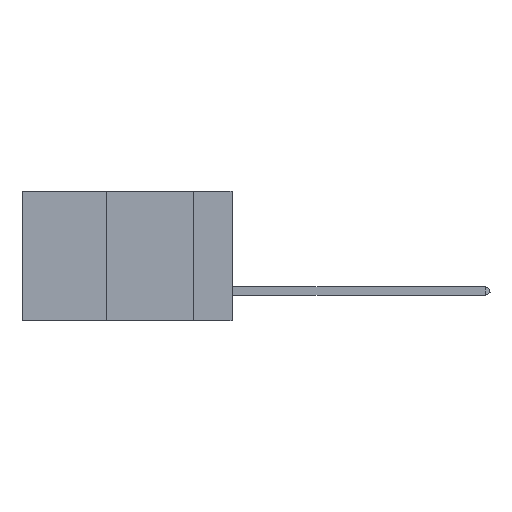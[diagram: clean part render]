
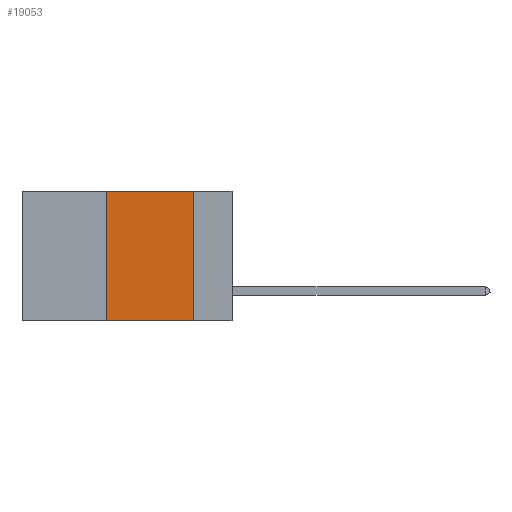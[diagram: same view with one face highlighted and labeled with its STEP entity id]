
A CAD part, left-side view. The second image highlights one B-rep face of the part: STEP entity #19053.
In plain terms, the highlighted planar face has unit normal (-1, 0, 0).
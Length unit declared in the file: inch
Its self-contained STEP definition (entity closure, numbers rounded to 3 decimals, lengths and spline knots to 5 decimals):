
#1876 = AXIS2_PLACEMENT_3D ( 'NONE', #14640, #10569, #2135 ) ;
#2042 = PLANE ( 'NONE',  #1876 ) ;
#2135 = DIRECTION ( 'NONE',  ( 0., 0., -1. ) ) ;
#3090 = LINE ( 'NONE', #6137, #24467 ) ;
#3694 = LINE ( 'NONE', #10751, #21509 ) ;
#4619 = ORIENTED_EDGE ( 'NONE', *, *, #13047, .T. ) ;
#5207 = LINE ( 'NONE', #14706, #13324 ) ;
#6137 = CARTESIAN_POINT ( 'NONE',  ( 0., 0.6, 0. ) ) ;
#8611 = EDGE_LOOP ( 'NONE', ( #18381, #15416, #20620, #4619 ) ) ;
#10569 = DIRECTION ( 'NONE',  ( 1., 0., 0. ) ) ;
#10751 = CARTESIAN_POINT ( 'NONE',  ( 0., 0.6, -0.37 ) ) ;
#11040 = VERTEX_POINT ( 'NONE', #12676 ) ;
#12396 = VECTOR ( 'NONE', #22250, 39.37008 ) ;
#12676 = CARTESIAN_POINT ( 'NONE',  ( 0., 0.36, 0. ) ) ;
#13047 = EDGE_CURVE ( 'NONE', #13778, #25661, #3694, .T. ) ;
#13324 = VECTOR ( 'NONE', #22996, 39.37008 ) ;
#13778 = VERTEX_POINT ( 'NONE', #18536 ) ;
#14640 = CARTESIAN_POINT ( 'NONE',  ( 0., 0.6, 0. ) ) ;
#14706 = CARTESIAN_POINT ( 'NONE',  ( 0., 0.11, 0. ) ) ;
#15001 = DIRECTION ( 'NONE',  ( 0., -1., 0. ) ) ;
#15416 = ORIENTED_EDGE ( 'NONE', *, *, #19083, .F. ) ;
#16041 = CARTESIAN_POINT ( 'NONE',  ( 0., 0.36, 0. ) ) ;
#16151 = VERTEX_POINT ( 'NONE', #24453 ) ;
#18381 = ORIENTED_EDGE ( 'NONE', *, *, #22425, .F. ) ;
#18536 = CARTESIAN_POINT ( 'NONE',  ( 0., 0.36, -0.37 ) ) ;
#18542 = LINE ( 'NONE', #16041, #12396 ) ;
#19053 = ADVANCED_FACE ( 'NONE', ( #25777 ), #2042, .F. ) ;
#19083 = EDGE_CURVE ( 'NONE', #11040, #16151, #3090, .T. ) ;
#20620 = ORIENTED_EDGE ( 'NONE', *, *, #21752, .F. ) ;
#21509 = VECTOR ( 'NONE', #15001, 39.37008 ) ;
#21752 = EDGE_CURVE ( 'NONE', #13778, #11040, #18542, .T. ) ;
#22250 = DIRECTION ( 'NONE',  ( 0., 0., 1. ) ) ;
#22425 = EDGE_CURVE ( 'NONE', #16151, #25661, #5207, .T. ) ;
#22996 = DIRECTION ( 'NONE',  ( 0., 0., -1. ) ) ;
#23015 = DIRECTION ( 'NONE',  ( 0., -1., 0. ) ) ;
#24453 = CARTESIAN_POINT ( 'NONE',  ( 0., 0.11, 0. ) ) ;
#24467 = VECTOR ( 'NONE', #23015, 39.37008 ) ;
#25661 = VERTEX_POINT ( 'NONE', #25855 ) ;
#25777 = FACE_OUTER_BOUND ( 'NONE', #8611, .T. ) ;
#25855 = CARTESIAN_POINT ( 'NONE',  ( 0., 0.11, -0.37 ) ) ;
